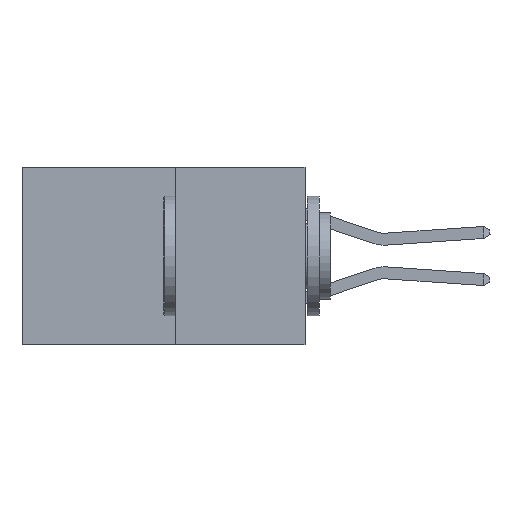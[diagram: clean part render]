
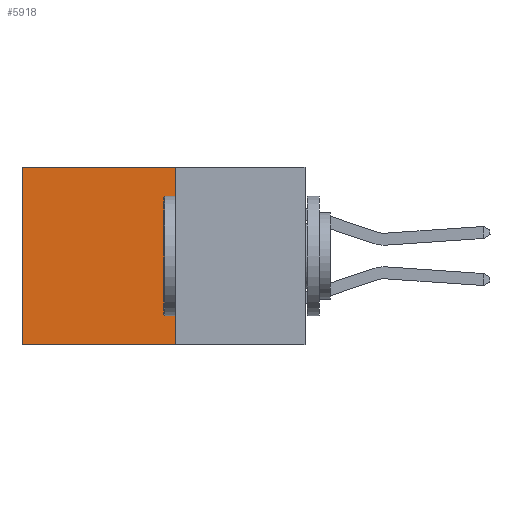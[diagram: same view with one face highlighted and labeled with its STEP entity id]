
A CAD part, left-side view. The second image highlights one B-rep face of the part: STEP entity #5918.
In plain terms, the highlighted planar face has unit normal (-1, 0, 0).
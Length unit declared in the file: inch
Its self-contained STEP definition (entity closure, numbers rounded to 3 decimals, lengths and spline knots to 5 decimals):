
#393 = EDGE_CURVE ( 'NONE', #5629, #4040, #7804, .T. ) ;
#575 = EDGE_CURVE ( 'NONE', #11712, #4040, #6071, .T. ) ;
#732 = CARTESIAN_POINT ( 'NONE',  ( 0.277, 0.59, -0.37 ) ) ;
#791 = VECTOR ( 'NONE', #12858, 39.37008 ) ;
#1187 = EDGE_CURVE ( 'NONE', #6581, #5629, #3648, .T. ) ;
#1762 = DIRECTION ( 'NONE',  ( 0., 0., -1. ) ) ;
#1903 = FACE_OUTER_BOUND ( 'NONE', #13233, .T. ) ;
#1917 = VECTOR ( 'NONE', #2068, 39.37008 ) ;
#2068 = DIRECTION ( 'NONE',  ( 0., 1., 0. ) ) ;
#2781 = EDGE_CURVE ( 'NONE', #6581, #11712, #10001, .T. ) ;
#2793 = ORIENTED_EDGE ( 'NONE', *, *, #1187, .F. ) ;
#2967 = CARTESIAN_POINT ( 'NONE',  ( 0.277, 0.27, 0. ) ) ;
#3648 = LINE ( 'NONE', #13985, #9854 ) ;
#4040 = VERTEX_POINT ( 'NONE', #4688 ) ;
#4688 = CARTESIAN_POINT ( 'NONE',  ( 0.277, 0.59, -0.37 ) ) ;
#4690 = ORIENTED_EDGE ( 'NONE', *, *, #393, .F. ) ;
#5371 = VECTOR ( 'NONE', #1762, 39.37008 ) ;
#5629 = VERTEX_POINT ( 'NONE', #13939 ) ;
#5918 = ADVANCED_FACE ( 'NONE', ( #1903 ), #12369, .F. ) ;
#6071 = LINE ( 'NONE', #732, #5371 ) ;
#6581 = VERTEX_POINT ( 'NONE', #7648 ) ;
#7648 = CARTESIAN_POINT ( 'NONE',  ( 0.277, 0.27, 0. ) ) ;
#7804 = LINE ( 'NONE', #13901, #1917 ) ;
#7935 = CARTESIAN_POINT ( 'NONE',  ( 0.277, 0.59, 0. ) ) ;
#9003 = ORIENTED_EDGE ( 'NONE', *, *, #2781, .T. ) ;
#9854 = VECTOR ( 'NONE', #10596, 39.37008 ) ;
#10001 = LINE ( 'NONE', #2967, #791 ) ;
#10596 = DIRECTION ( 'NONE',  ( 0., 0., -1. ) ) ;
#11712 = VERTEX_POINT ( 'NONE', #7935 ) ;
#12135 = ORIENTED_EDGE ( 'NONE', *, *, #575, .T. ) ;
#12337 = DIRECTION ( 'NONE',  ( 0., 0., -1. ) ) ;
#12346 = DIRECTION ( 'NONE',  ( 1., 0., 0. ) ) ;
#12369 = PLANE ( 'NONE',  #12552 ) ;
#12434 = CARTESIAN_POINT ( 'NONE',  ( 0.277, 0.27, -0.37 ) ) ;
#12552 = AXIS2_PLACEMENT_3D ( 'NONE', #12434, #12346, #12337 ) ;
#12858 = DIRECTION ( 'NONE',  ( 0., 1., 0. ) ) ;
#13233 = EDGE_LOOP ( 'NONE', ( #12135, #4690, #2793, #9003 ) ) ;
#13901 = CARTESIAN_POINT ( 'NONE',  ( 0.277, 0.27, -0.37 ) ) ;
#13939 = CARTESIAN_POINT ( 'NONE',  ( 0.277, 0.27, -0.37 ) ) ;
#13985 = CARTESIAN_POINT ( 'NONE',  ( 0.277, 0.27, -0.37 ) ) ;
